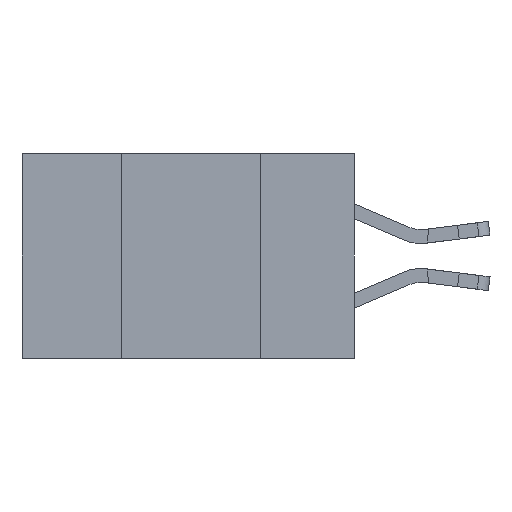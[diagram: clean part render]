
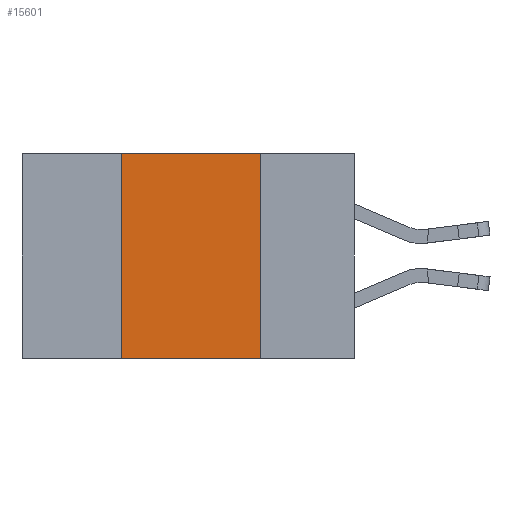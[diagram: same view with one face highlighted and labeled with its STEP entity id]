
A CAD part, left-side view. The second image highlights one B-rep face of the part: STEP entity #15601.
In plain terms, the highlighted planar face has unit normal (-1, 0, 0).
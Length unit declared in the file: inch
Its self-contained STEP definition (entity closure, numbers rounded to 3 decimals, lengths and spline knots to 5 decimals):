
#1365 = LINE ( 'NONE', #2423, #7602 ) ;
#1548 = DIRECTION ( 'NONE',  ( 1., 0., 0. ) ) ;
#1918 = LINE ( 'NONE', #14891, #14201 ) ;
#2423 = CARTESIAN_POINT ( 'NONE',  ( 0., 0.42, -0.37 ) ) ;
#2916 = EDGE_LOOP ( 'NONE', ( #14343, #5395, #8055, #15039 ) ) ;
#3071 = LINE ( 'NONE', #11843, #15607 ) ;
#3239 = DIRECTION ( 'NONE',  ( 0., -1., 0. ) ) ;
#4467 = AXIS2_PLACEMENT_3D ( 'NONE', #9011, #1548, #10240 ) ;
#5242 = VERTEX_POINT ( 'NONE', #6459 ) ;
#5395 = ORIENTED_EDGE ( 'NONE', *, *, #12265, .F. ) ;
#6237 = DIRECTION ( 'NONE',  ( 0., -1., 0. ) ) ;
#6459 = CARTESIAN_POINT ( 'NONE',  ( 0., 0.42, 0. ) ) ;
#6600 = VECTOR ( 'NONE', #6237, 39.37008 ) ;
#7347 = DIRECTION ( 'NONE',  ( 0., 0., 1. ) ) ;
#7602 = VECTOR ( 'NONE', #7347, 39.37008 ) ;
#8055 = ORIENTED_EDGE ( 'NONE', *, *, #13074, .F. ) ;
#8865 = CARTESIAN_POINT ( 'NONE',  ( 0., 0.17, -0.37 ) ) ;
#8898 = VERTEX_POINT ( 'NONE', #13924 ) ;
#9011 = CARTESIAN_POINT ( 'NONE',  ( 0., 0.6, 0. ) ) ;
#9994 = CARTESIAN_POINT ( 'NONE',  ( 0., 0.6, -0.37 ) ) ;
#10240 = DIRECTION ( 'NONE',  ( 0., 0., -1. ) ) ;
#10397 = CARTESIAN_POINT ( 'NONE',  ( 0., 0.17, 0. ) ) ;
#10442 = VERTEX_POINT ( 'NONE', #10397 ) ;
#10962 = FACE_OUTER_BOUND ( 'NONE', #2916, .T. ) ;
#11382 = PLANE ( 'NONE',  #4467 ) ;
#11439 = EDGE_CURVE ( 'NONE', #10442, #15302, #1918, .T. ) ;
#11843 = CARTESIAN_POINT ( 'NONE',  ( 0., 0.6, 0. ) ) ;
#12265 = EDGE_CURVE ( 'NONE', #5242, #10442, #3071, .T. ) ;
#13074 = EDGE_CURVE ( 'NONE', #8898, #5242, #1365, .T. ) ;
#13731 = DIRECTION ( 'NONE',  ( 0., 0., -1. ) ) ;
#13872 = EDGE_CURVE ( 'NONE', #8898, #15302, #15828, .T. ) ;
#13924 = CARTESIAN_POINT ( 'NONE',  ( 0., 0.42, -0.37 ) ) ;
#14201 = VECTOR ( 'NONE', #13731, 39.37008 ) ;
#14343 = ORIENTED_EDGE ( 'NONE', *, *, #11439, .F. ) ;
#14891 = CARTESIAN_POINT ( 'NONE',  ( 0., 0.17, -0.37 ) ) ;
#15039 = ORIENTED_EDGE ( 'NONE', *, *, #13872, .T. ) ;
#15302 = VERTEX_POINT ( 'NONE', #8865 ) ;
#15601 = ADVANCED_FACE ( 'NONE', ( #10962 ), #11382, .F. ) ;
#15607 = VECTOR ( 'NONE', #3239, 39.37008 ) ;
#15828 = LINE ( 'NONE', #9994, #6600 ) ;
